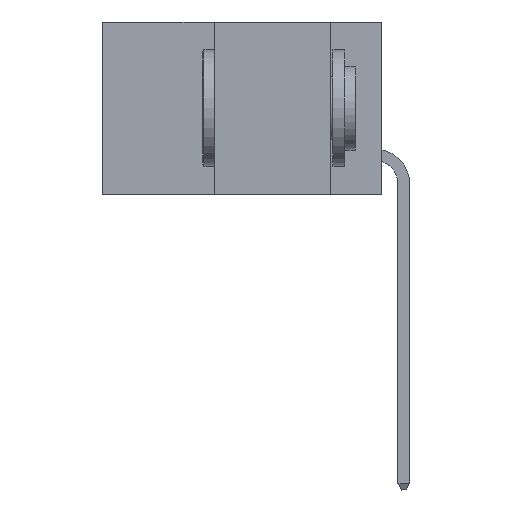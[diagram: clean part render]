
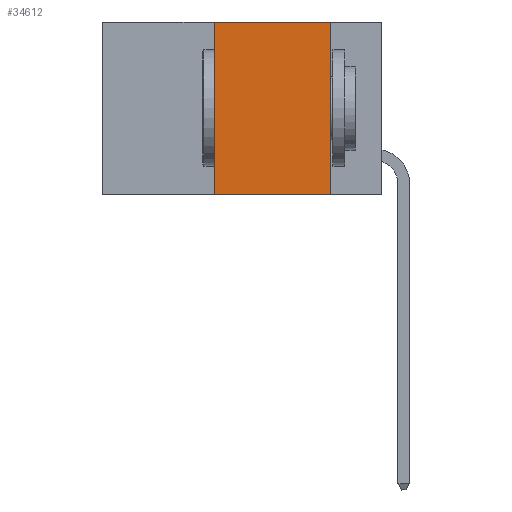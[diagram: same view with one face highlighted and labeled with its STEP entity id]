
A CAD part, left-side view. The second image highlights one B-rep face of the part: STEP entity #34612.
In plain terms, the highlighted planar face has unit normal (-1, 0, 0).
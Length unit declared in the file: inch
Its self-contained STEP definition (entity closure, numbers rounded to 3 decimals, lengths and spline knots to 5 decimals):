
#748 = VECTOR ( 'NONE', #45100, 39.37008 ) ;
#1370 = LINE ( 'NONE', #43467, #41128 ) ;
#3319 = CARTESIAN_POINT ( 'NONE',  ( 0., 0.6, 0. ) ) ;
#5344 = DIRECTION ( 'NONE',  ( 0., -1., 0. ) ) ;
#6450 = VERTEX_POINT ( 'NONE', #26546 ) ;
#8916 = LINE ( 'NONE', #49452, #12502 ) ;
#9767 = CARTESIAN_POINT ( 'NONE',  ( 0., 0.11, 0. ) ) ;
#11278 = VECTOR ( 'NONE', #35695, 39.37008 ) ;
#12502 = VECTOR ( 'NONE', #34971, 39.37008 ) ;
#16295 = AXIS2_PLACEMENT_3D ( 'NONE', #3319, #41450, #18259 ) ;
#18259 = DIRECTION ( 'NONE',  ( 0., 0., -1. ) ) ;
#18393 = ORIENTED_EDGE ( 'NONE', *, *, #37188, .F. ) ;
#20069 = EDGE_LOOP ( 'NONE', ( #18393, #42505, #40367, #25997 ) ) ;
#21220 = LINE ( 'NONE', #40936, #748 ) ;
#23030 = FACE_OUTER_BOUND ( 'NONE', #20069, .T. ) ;
#23251 = CARTESIAN_POINT ( 'NONE',  ( 0., 0.36, 0. ) ) ;
#23992 = VERTEX_POINT ( 'NONE', #45747 ) ;
#25997 = ORIENTED_EDGE ( 'NONE', *, *, #49614, .T. ) ;
#26546 = CARTESIAN_POINT ( 'NONE',  ( 0., 0.11, -0.37 ) ) ;
#26969 = EDGE_CURVE ( 'NONE', #23992, #47268, #8916, .T. ) ;
#31024 = PLANE ( 'NONE',  #16295 ) ;
#34612 = ADVANCED_FACE ( 'NONE', ( #23030 ), #31024, .F. ) ;
#34971 = DIRECTION ( 'NONE',  ( 0., 0., 1. ) ) ;
#35522 = CARTESIAN_POINT ( 'NONE',  ( 0., 0.11, 0. ) ) ;
#35695 = DIRECTION ( 'NONE',  ( 0., 0., -1. ) ) ;
#37188 = EDGE_CURVE ( 'NONE', #47440, #6450, #43758, .T. ) ;
#40367 = ORIENTED_EDGE ( 'NONE', *, *, #26969, .F. ) ;
#40936 = CARTESIAN_POINT ( 'NONE',  ( 0., 0.6, 0. ) ) ;
#41128 = VECTOR ( 'NONE', #5344, 39.37008 ) ;
#41450 = DIRECTION ( 'NONE',  ( 1., 0., 0. ) ) ;
#42505 = ORIENTED_EDGE ( 'NONE', *, *, #44874, .F. ) ;
#43467 = CARTESIAN_POINT ( 'NONE',  ( 0., 0.6, -0.37 ) ) ;
#43758 = LINE ( 'NONE', #35522, #11278 ) ;
#44874 = EDGE_CURVE ( 'NONE', #47268, #47440, #21220, .T. ) ;
#45100 = DIRECTION ( 'NONE',  ( 0., -1., 0. ) ) ;
#45747 = CARTESIAN_POINT ( 'NONE',  ( 0., 0.36, -0.37 ) ) ;
#47268 = VERTEX_POINT ( 'NONE', #23251 ) ;
#47440 = VERTEX_POINT ( 'NONE', #9767 ) ;
#49452 = CARTESIAN_POINT ( 'NONE',  ( 0., 0.36, 0. ) ) ;
#49614 = EDGE_CURVE ( 'NONE', #23992, #6450, #1370, .T. ) ;
